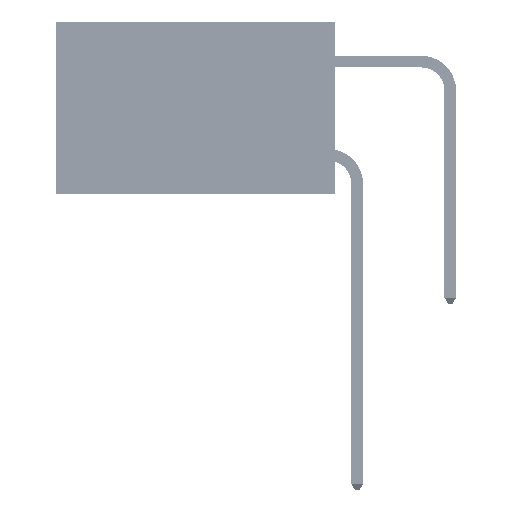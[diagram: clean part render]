
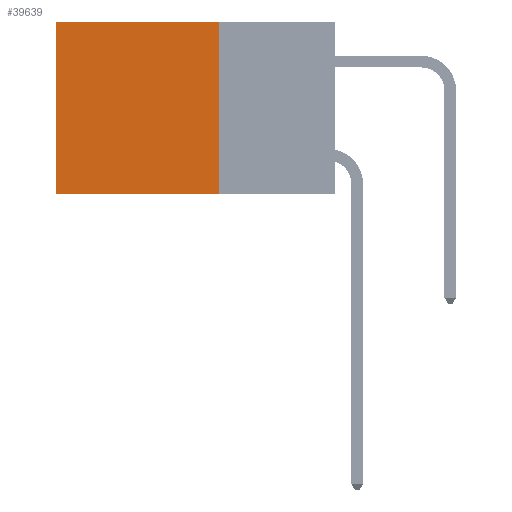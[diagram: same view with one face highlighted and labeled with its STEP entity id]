
A CAD part, left-side view. The second image highlights one B-rep face of the part: STEP entity #39639.
In plain terms, the highlighted planar face has unit normal (-1, 0, 0).
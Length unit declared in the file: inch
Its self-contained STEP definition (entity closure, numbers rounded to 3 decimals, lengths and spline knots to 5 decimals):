
#49 = VECTOR ( 'NONE', #9681, 39.37008 ) ;
#747 = EDGE_CURVE ( 'NONE', #22804, #17821, #7259, .T. ) ;
#1883 = EDGE_CURVE ( 'NONE', #33917, #20966, #5611, .T. ) ;
#2669 = DIRECTION ( 'NONE',  ( 0., 1., 0. ) ) ;
#3431 = LINE ( 'NONE', #30007, #24395 ) ;
#5611 = LINE ( 'NONE', #16249, #9467 ) ;
#7259 = LINE ( 'NONE', #42716, #22261 ) ;
#7352 = DIRECTION ( 'NONE',  ( 0., 1., 0. ) ) ;
#8493 = CARTESIAN_POINT ( 'NONE',  ( 0.2875, 0.25, -0.37 ) ) ;
#9467 = VECTOR ( 'NONE', #2669, 39.37008 ) ;
#9681 = DIRECTION ( 'NONE',  ( 0., 0., -1. ) ) ;
#10324 = ORIENTED_EDGE ( 'NONE', *, *, #37357, .F. ) ;
#11310 = ORIENTED_EDGE ( 'NONE', *, *, #38512, .T. ) ;
#11529 = CARTESIAN_POINT ( 'NONE',  ( 0.2875, 0.25, 0. ) ) ;
#11795 = EDGE_LOOP ( 'NONE', ( #11310, #15636, #10324, #40464 ) ) ;
#14392 = CARTESIAN_POINT ( 'NONE',  ( 0.2875, 0.6, 0. ) ) ;
#15636 = ORIENTED_EDGE ( 'NONE', *, *, #1883, .F. ) ;
#16249 = CARTESIAN_POINT ( 'NONE',  ( 0.2875, 0.25, -0.37 ) ) ;
#17821 = VERTEX_POINT ( 'NONE', #14392 ) ;
#19373 = AXIS2_PLACEMENT_3D ( 'NONE', #30036, #23253, #26471 ) ;
#20966 = VERTEX_POINT ( 'NONE', #34791 ) ;
#22115 = LINE ( 'NONE', #44866, #49 ) ;
#22261 = VECTOR ( 'NONE', #7352, 39.37008 ) ;
#22804 = VERTEX_POINT ( 'NONE', #11529 ) ;
#23253 = DIRECTION ( 'NONE',  ( 1., 0., 0. ) ) ;
#24395 = VECTOR ( 'NONE', #40819, 39.37008 ) ;
#26471 = DIRECTION ( 'NONE',  ( 0., 0., -1. ) ) ;
#27034 = FACE_OUTER_BOUND ( 'NONE', #11795, .T. ) ;
#30007 = CARTESIAN_POINT ( 'NONE',  ( 0.2875, 0.25, 0. ) ) ;
#30036 = CARTESIAN_POINT ( 'NONE',  ( 0.2875, 0.25, 0. ) ) ;
#33917 = VERTEX_POINT ( 'NONE', #8493 ) ;
#34791 = CARTESIAN_POINT ( 'NONE',  ( 0.2875, 0.6, -0.37 ) ) ;
#37357 = EDGE_CURVE ( 'NONE', #22804, #33917, #3431, .T. ) ;
#38512 = EDGE_CURVE ( 'NONE', #17821, #20966, #22115, .T. ) ;
#39639 = ADVANCED_FACE ( 'NONE', ( #27034 ), #44396, .F. ) ;
#40464 = ORIENTED_EDGE ( 'NONE', *, *, #747, .T. ) ;
#40819 = DIRECTION ( 'NONE',  ( 0., 0., -1. ) ) ;
#42716 = CARTESIAN_POINT ( 'NONE',  ( 0.2875, 0.25, 0. ) ) ;
#44396 = PLANE ( 'NONE',  #19373 ) ;
#44866 = CARTESIAN_POINT ( 'NONE',  ( 0.2875, 0.6, 0. ) ) ;
